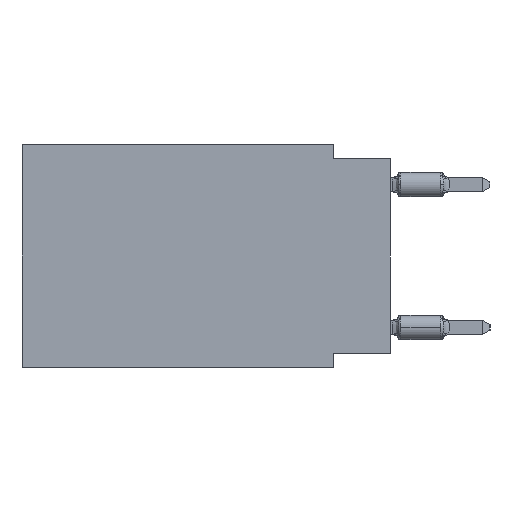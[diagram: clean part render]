
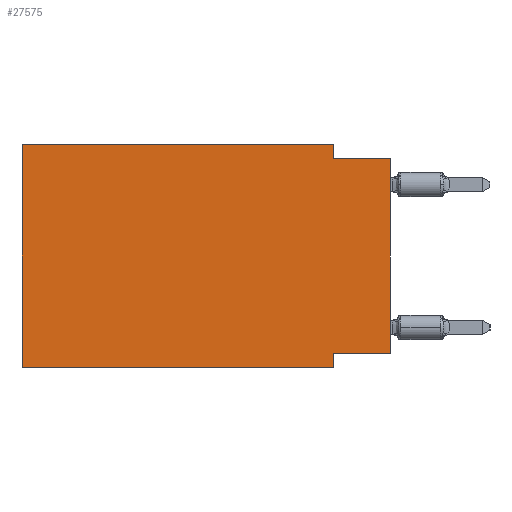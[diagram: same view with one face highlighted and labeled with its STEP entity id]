
A CAD part, left-side view. The second image highlights one B-rep face of the part: STEP entity #27575.
In plain terms, the highlighted planar face has unit normal (-1, 0, 0).
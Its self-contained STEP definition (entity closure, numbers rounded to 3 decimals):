
#1134 = LINE ( 'NONE', #6638, #23663 ) ;
#1149 = VECTOR ( 'NONE', #4797, 1000. ) ;
#2035 = CARTESIAN_POINT ( 'NONE',  ( 0., 0., 0. ) ) ;
#2383 = FACE_OUTER_BOUND ( 'NONE', #16456, .T. ) ;
#2545 = DIRECTION ( 'NONE',  ( 0., 0., -1. ) ) ;
#3368 = VECTOR ( 'NONE', #26401, 1000. ) ;
#3497 = CARTESIAN_POINT ( 'NONE',  ( 0., 16.383, -9.906 ) ) ;
#4342 = ORIENTED_EDGE ( 'NONE', *, *, #5710, .F. ) ;
#4797 = DIRECTION ( 'NONE',  ( 0., -1., 0. ) ) ;
#4910 = VERTEX_POINT ( 'NONE', #27140 ) ;
#5448 = CARTESIAN_POINT ( 'NONE',  ( 0., 16.383, 0. ) ) ;
#5710 = EDGE_CURVE ( 'NONE', #21367, #28030, #22152, .T. ) ;
#6120 = VECTOR ( 'NONE', #9945, 1000. ) ;
#6131 = DIRECTION ( 'NONE',  ( 0., 1., 0. ) ) ;
#6638 = CARTESIAN_POINT ( 'NONE',  ( 0., 0., -9.271 ) ) ;
#7239 = VECTOR ( 'NONE', #26695, 1000. ) ;
#8006 = LINE ( 'NONE', #29455, #26886 ) ;
#8696 = CARTESIAN_POINT ( 'NONE',  ( 0., 2.54, -0.635 ) ) ;
#8823 = LINE ( 'NONE', #3497, #7239 ) ;
#9451 = CARTESIAN_POINT ( 'NONE',  ( 0., 0., -9.271 ) ) ;
#9614 = CARTESIAN_POINT ( 'NONE',  ( 0., 0., -0.635 ) ) ;
#9784 = CARTESIAN_POINT ( 'NONE',  ( 0., 16.383, 0. ) ) ;
#9866 = CARTESIAN_POINT ( 'NONE',  ( 0., 0., -0.635 ) ) ;
#9945 = DIRECTION ( 'NONE',  ( 0., 0., 1. ) ) ;
#10020 = EDGE_CURVE ( 'NONE', #4910, #13001, #8006, .T. ) ;
#10971 = ORIENTED_EDGE ( 'NONE', *, *, #25166, .T. ) ;
#11195 = CARTESIAN_POINT ( 'NONE',  ( 0., 2.54, -9.271 ) ) ;
#11467 = VERTEX_POINT ( 'NONE', #9866 ) ;
#12881 = CARTESIAN_POINT ( 'NONE',  ( 0., 16.383, 0. ) ) ;
#13001 = VERTEX_POINT ( 'NONE', #8696 ) ;
#14096 = VERTEX_POINT ( 'NONE', #32291 ) ;
#14285 = EDGE_CURVE ( 'NONE', #13001, #11467, #33153, .T. ) ;
#14344 = EDGE_CURVE ( 'NONE', #14096, #4910, #28492, .T. ) ;
#14513 = CARTESIAN_POINT ( 'NONE',  ( 0., 16.383, -9.906 ) ) ;
#14627 = EDGE_CURVE ( 'NONE', #21643, #21367, #1134, .T. ) ;
#14751 = LINE ( 'NONE', #2035, #6120 ) ;
#14892 = ORIENTED_EDGE ( 'NONE', *, *, #14285, .F. ) ;
#15942 = AXIS2_PLACEMENT_3D ( 'NONE', #12881, #20756, #2545 ) ;
#16456 = EDGE_LOOP ( 'NONE', ( #21664, #14892, #26654, #17650, #32800, #10971, #4342, #21421 ) ) ;
#17246 = CARTESIAN_POINT ( 'NONE',  ( 0., 2.54, -9.906 ) ) ;
#17650 = ORIENTED_EDGE ( 'NONE', *, *, #14344, .F. ) ;
#18349 = PLANE ( 'NONE',  #15942 ) ;
#18869 = VECTOR ( 'NONE', #29892, 1000. ) ;
#20079 = DIRECTION ( 'NONE',  ( 0., -1., 0. ) ) ;
#20756 = DIRECTION ( 'NONE',  ( 1., 0., 0. ) ) ;
#21367 = VERTEX_POINT ( 'NONE', #11195 ) ;
#21421 = ORIENTED_EDGE ( 'NONE', *, *, #14627, .F. ) ;
#21643 = VERTEX_POINT ( 'NONE', #9451 ) ;
#21664 = ORIENTED_EDGE ( 'NONE', *, *, #27371, .T. ) ;
#22152 = LINE ( 'NONE', #24396, #18869 ) ;
#23663 = VECTOR ( 'NONE', #6131, 1000. ) ;
#24396 = CARTESIAN_POINT ( 'NONE',  ( 0., 2.54, -9.906 ) ) ;
#25166 = EDGE_CURVE ( 'NONE', #32736, #28030, #8823, .T. ) ;
#25852 = VECTOR ( 'NONE', #20079, 1000. ) ;
#26036 = DIRECTION ( 'NONE',  ( 0., 0., -1. ) ) ;
#26401 = DIRECTION ( 'NONE',  ( 0., 0., 1. ) ) ;
#26654 = ORIENTED_EDGE ( 'NONE', *, *, #10020, .F. ) ;
#26695 = DIRECTION ( 'NONE',  ( 0., -1., 0. ) ) ;
#26886 = VECTOR ( 'NONE', #26036, 1000. ) ;
#27140 = CARTESIAN_POINT ( 'NONE',  ( 0., 2.54, 0. ) ) ;
#27371 = EDGE_CURVE ( 'NONE', #21643, #11467, #14751, .T. ) ;
#27575 = ADVANCED_FACE ( 'NONE', ( #2383 ), #18349, .F. ) ;
#28030 = VERTEX_POINT ( 'NONE', #17246 ) ;
#28492 = LINE ( 'NONE', #9784, #1149 ) ;
#28988 = LINE ( 'NONE', #5448, #3368 ) ;
#29455 = CARTESIAN_POINT ( 'NONE',  ( 0., 2.54, 0. ) ) ;
#29892 = DIRECTION ( 'NONE',  ( 0., 0., -1. ) ) ;
#31131 = EDGE_CURVE ( 'NONE', #32736, #14096, #28988, .T. ) ;
#32291 = CARTESIAN_POINT ( 'NONE',  ( 0., 16.383, 0. ) ) ;
#32736 = VERTEX_POINT ( 'NONE', #14513 ) ;
#32800 = ORIENTED_EDGE ( 'NONE', *, *, #31131, .F. ) ;
#33153 = LINE ( 'NONE', #9614, #25852 ) ;
